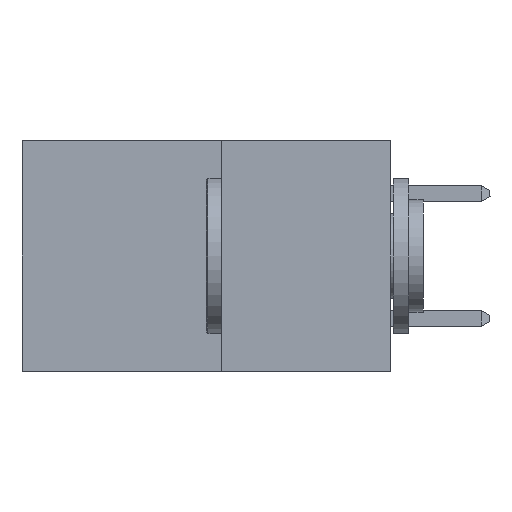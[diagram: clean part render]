
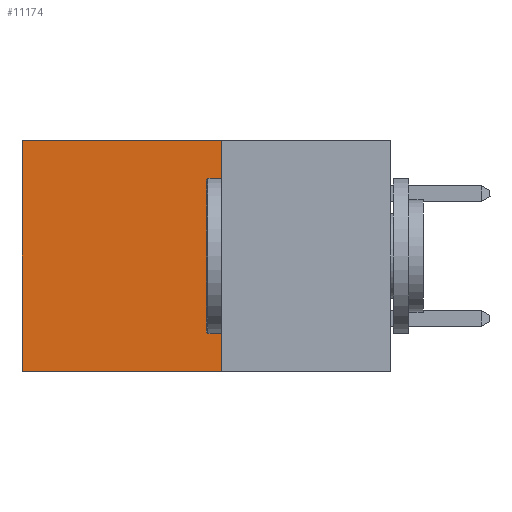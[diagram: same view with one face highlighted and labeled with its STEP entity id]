
A CAD part, left-side view. The second image highlights one B-rep face of the part: STEP entity #11174.
In plain terms, the highlighted planar face has unit normal (-1, 0, 0).
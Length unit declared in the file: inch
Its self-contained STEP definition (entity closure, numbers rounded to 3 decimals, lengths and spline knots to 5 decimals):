
#192 = CARTESIAN_POINT ( 'NONE',  ( 0.277, 0.27, -0.37 ) ) ;
#895 = LINE ( 'NONE', #5780, #16337 ) ;
#2547 = EDGE_CURVE ( 'NONE', #5652, #3354, #11209, .T. ) ;
#3354 = VERTEX_POINT ( 'NONE', #17798 ) ;
#3460 = DIRECTION ( 'NONE',  ( 0., 0., -1. ) ) ;
#4776 = LINE ( 'NONE', #7502, #16163 ) ;
#5045 = EDGE_CURVE ( 'NONE', #12623, #5652, #895, .T. ) ;
#5566 = CARTESIAN_POINT ( 'NONE',  ( 0.277, 0.59, 0. ) ) ;
#5639 = ORIENTED_EDGE ( 'NONE', *, *, #5045, .T. ) ;
#5652 = VERTEX_POINT ( 'NONE', #5566 ) ;
#5780 = CARTESIAN_POINT ( 'NONE',  ( 0.277, 0.27, 0. ) ) ;
#7005 = EDGE_LOOP ( 'NONE', ( #16063, #15635, #7716, #5639 ) ) ;
#7301 = VECTOR ( 'NONE', #12265, 39.37008 ) ;
#7309 = DIRECTION ( 'NONE',  ( 0., 1., 0. ) ) ;
#7423 = FACE_OUTER_BOUND ( 'NONE', #7005, .T. ) ;
#7502 = CARTESIAN_POINT ( 'NONE',  ( 0.277, 0.27, -0.37 ) ) ;
#7716 = ORIENTED_EDGE ( 'NONE', *, *, #11822, .F. ) ;
#7883 = VERTEX_POINT ( 'NONE', #192 ) ;
#8853 = AXIS2_PLACEMENT_3D ( 'NONE', #18804, #18764, #19138 ) ;
#9199 = PLANE ( 'NONE',  #8853 ) ;
#9710 = CARTESIAN_POINT ( 'NONE',  ( 0.277, 0.27, 0. ) ) ;
#11174 = ADVANCED_FACE ( 'NONE', ( #7423 ), #9199, .F. ) ;
#11209 = LINE ( 'NONE', #11964, #7301 ) ;
#11822 = EDGE_CURVE ( 'NONE', #12623, #7883, #15280, .T. ) ;
#11964 = CARTESIAN_POINT ( 'NONE',  ( 0.277, 0.59, -0.37 ) ) ;
#12265 = DIRECTION ( 'NONE',  ( 0., 0., -1. ) ) ;
#12623 = VERTEX_POINT ( 'NONE', #9710 ) ;
#12720 = EDGE_CURVE ( 'NONE', #7883, #3354, #4776, .T. ) ;
#13143 = DIRECTION ( 'NONE',  ( 0., 1., 0. ) ) ;
#13980 = CARTESIAN_POINT ( 'NONE',  ( 0.277, 0.27, -0.37 ) ) ;
#15280 = LINE ( 'NONE', #13980, #19230 ) ;
#15635 = ORIENTED_EDGE ( 'NONE', *, *, #12720, .F. ) ;
#16063 = ORIENTED_EDGE ( 'NONE', *, *, #2547, .T. ) ;
#16163 = VECTOR ( 'NONE', #7309, 39.37008 ) ;
#16337 = VECTOR ( 'NONE', #13143, 39.37008 ) ;
#17798 = CARTESIAN_POINT ( 'NONE',  ( 0.277, 0.59, -0.37 ) ) ;
#18764 = DIRECTION ( 'NONE',  ( 1., 0., 0. ) ) ;
#18804 = CARTESIAN_POINT ( 'NONE',  ( 0.277, 0.27, -0.37 ) ) ;
#19138 = DIRECTION ( 'NONE',  ( 0., 0., -1. ) ) ;
#19230 = VECTOR ( 'NONE', #3460, 39.37008 ) ;
